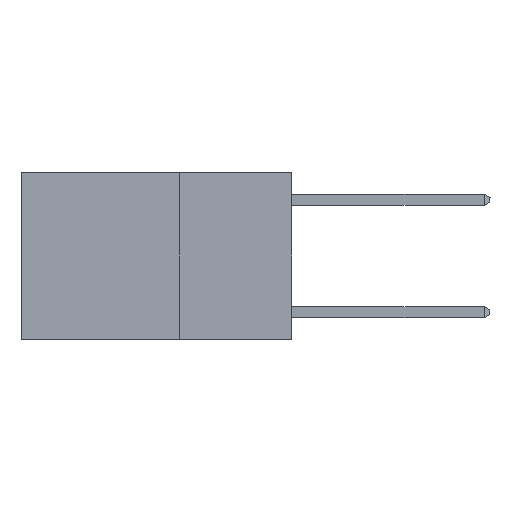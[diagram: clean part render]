
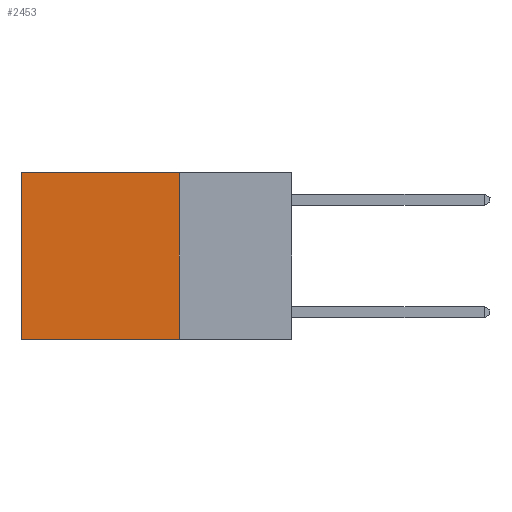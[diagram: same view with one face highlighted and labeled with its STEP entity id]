
A CAD part, left-side view. The second image highlights one B-rep face of the part: STEP entity #2453.
In plain terms, the highlighted planar face has unit normal (-1, 0, 0).
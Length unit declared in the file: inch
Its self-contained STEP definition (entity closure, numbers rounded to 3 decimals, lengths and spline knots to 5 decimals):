
#158 = ORIENTED_EDGE ( 'NONE', *, *, #6785, .F. ) ;
#707 = VECTOR ( 'NONE', #6495, 39.37008 ) ;
#928 = LINE ( 'NONE', #1331, #6851 ) ;
#1061 = LINE ( 'NONE', #7604, #707 ) ;
#1079 = CARTESIAN_POINT ( 'NONE',  ( 0.2625, 0.25, 0. ) ) ;
#1331 = CARTESIAN_POINT ( 'NONE',  ( 0.2625, 0.25, 0. ) ) ;
#1379 = DIRECTION ( 'NONE',  ( 0., 1., 0. ) ) ;
#1633 = CARTESIAN_POINT ( 'NONE',  ( 0.2625, 0.25, -0.37 ) ) ;
#2432 = LINE ( 'NONE', #5735, #10660 ) ;
#2437 = VERTEX_POINT ( 'NONE', #1079 ) ;
#2453 = ADVANCED_FACE ( 'NONE', ( #6654 ), #8020, .F. ) ;
#2820 = CARTESIAN_POINT ( 'NONE',  ( 0.2625, 0.6, -0.37 ) ) ;
#3361 = ORIENTED_EDGE ( 'NONE', *, *, #12770, .T. ) ;
#3454 = AXIS2_PLACEMENT_3D ( 'NONE', #13739, #8490, #6238 ) ;
#3575 = ORIENTED_EDGE ( 'NONE', *, *, #11984, .T. ) ;
#4179 = ORIENTED_EDGE ( 'NONE', *, *, #6806, .F. ) ;
#5322 = VERTEX_POINT ( 'NONE', #13259 ) ;
#5735 = CARTESIAN_POINT ( 'NONE',  ( 0.2625, 0.25, 0. ) ) ;
#5805 = CARTESIAN_POINT ( 'NONE',  ( 0.2625, 0.25, -0.37 ) ) ;
#6238 = DIRECTION ( 'NONE',  ( 0., 0., -1. ) ) ;
#6380 = VERTEX_POINT ( 'NONE', #1633 ) ;
#6495 = DIRECTION ( 'NONE',  ( 0., 0., -1. ) ) ;
#6654 = FACE_OUTER_BOUND ( 'NONE', #11580, .T. ) ;
#6785 = EDGE_CURVE ( 'NONE', #2437, #6380, #928, .T. ) ;
#6806 = EDGE_CURVE ( 'NONE', #6380, #8971, #12140, .T. ) ;
#6851 = VECTOR ( 'NONE', #12529, 39.37008 ) ;
#7604 = CARTESIAN_POINT ( 'NONE',  ( 0.2625, 0.6, 0. ) ) ;
#8020 = PLANE ( 'NONE',  #3454 ) ;
#8490 = DIRECTION ( 'NONE',  ( 1., 0., 0. ) ) ;
#8971 = VERTEX_POINT ( 'NONE', #2820 ) ;
#9132 = VECTOR ( 'NONE', #1379, 39.37008 ) ;
#10250 = DIRECTION ( 'NONE',  ( 0., 1., 0. ) ) ;
#10660 = VECTOR ( 'NONE', #10250, 39.37008 ) ;
#11580 = EDGE_LOOP ( 'NONE', ( #3575, #4179, #158, #3361 ) ) ;
#11984 = EDGE_CURVE ( 'NONE', #5322, #8971, #1061, .T. ) ;
#12140 = LINE ( 'NONE', #5805, #9132 ) ;
#12529 = DIRECTION ( 'NONE',  ( 0., 0., -1. ) ) ;
#12770 = EDGE_CURVE ( 'NONE', #2437, #5322, #2432, .T. ) ;
#13259 = CARTESIAN_POINT ( 'NONE',  ( 0.2625, 0.6, 0. ) ) ;
#13739 = CARTESIAN_POINT ( 'NONE',  ( 0.2625, 0.25, 0. ) ) ;
